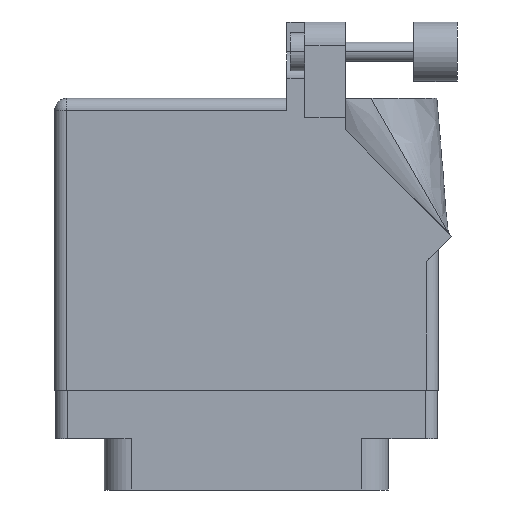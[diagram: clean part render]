
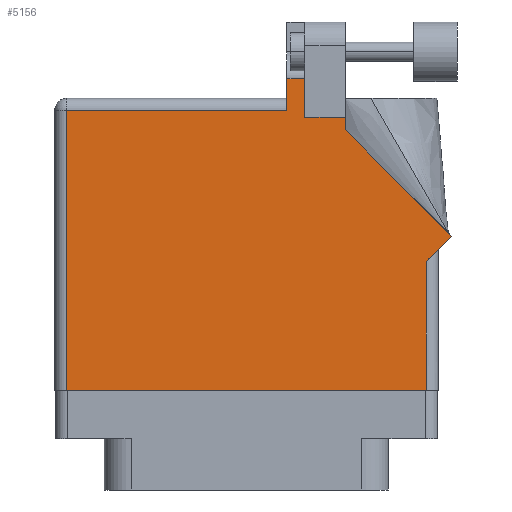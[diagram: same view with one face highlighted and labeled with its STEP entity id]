
A CAD part, front view. The second image highlights one B-rep face of the part: STEP entity #5156.
In plain terms, the highlighted face is planar.
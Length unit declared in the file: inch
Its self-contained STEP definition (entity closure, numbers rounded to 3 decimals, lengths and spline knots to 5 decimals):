
#82 = VECTOR ( 'NONE', #22160, 39.37008 ) ;
#381 = CARTESIAN_POINT ( 'NONE',  ( 0.519, 1.26442, 0.455 ) ) ;
#1623 = LINE ( 'NONE', #15452, #34094 ) ;
#1625 = CARTESIAN_POINT ( 'NONE',  ( 0.63677, 1.5315, 0.455 ) ) ;
#1646 = VECTOR ( 'NONE', #5734, 39.37008 ) ;
#2080 = VECTOR ( 'NONE', #26862, 39.37008 ) ;
#2097 = LINE ( 'NONE', #30293, #11346 ) ;
#2348 = ORIENTED_EDGE ( 'NONE', *, *, #28803, .T. ) ;
#2803 = VECTOR ( 'NONE', #6872, 39.37008 ) ;
#3260 = VECTOR ( 'NONE', #18487, 39.37008 ) ;
#3266 = VECTOR ( 'NONE', #21904, 39.37008 ) ;
#4062 = VERTEX_POINT ( 'NONE', #29323 ) ;
#4336 = VERTEX_POINT ( 'NONE', #22237 ) ;
#4407 = VERTEX_POINT ( 'NONE', #17761 ) ;
#4456 = EDGE_CURVE ( 'NONE', #25277, #4407, #30085, .T. ) ;
#4702 = ORIENTED_EDGE ( 'NONE', *, *, #26649, .T. ) ;
#5156 = ADVANCED_FACE ( 'NONE', ( #26941 ), #23604, .F. ) ;
#5289 = VERTEX_POINT ( 'NONE', #10062 ) ;
#5734 = DIRECTION ( 'NONE',  ( 0., -1., 0. ) ) ;
#6723 = DIRECTION ( 'NONE',  ( 0., 0., -1. ) ) ;
#6872 = DIRECTION ( 'NONE',  ( 0., 1., 0. ) ) ;
#6888 = LINE ( 'NONE', #381, #25368 ) ;
#7732 = EDGE_CURVE ( 'NONE', #17834, #10180, #15529, .T. ) ;
#8005 = VECTOR ( 'NONE', #28396, 39.37008 ) ;
#9336 = LINE ( 'NONE', #16384, #82 ) ;
#9558 = LINE ( 'NONE', #18669, #2080 ) ;
#9890 = EDGE_CURVE ( 'NONE', #10180, #23784, #9558, .T. ) ;
#10062 = CARTESIAN_POINT ( 'NONE',  ( 0.519, 1.26442, 0.455 ) ) ;
#10123 = EDGE_CURVE ( 'NONE', #23784, #4336, #25384, .T. ) ;
#10180 = VERTEX_POINT ( 'NONE', #11519 ) ;
#10313 = ORIENTED_EDGE ( 'NONE', *, *, #14590, .T. ) ;
#11346 = VECTOR ( 'NONE', #13627, 39.37008 ) ;
#11415 = VERTEX_POINT ( 'NONE', #34351 ) ;
#11519 = CARTESIAN_POINT ( 'NONE',  ( 0.212, 1.368, 0.455 ) ) ;
#12117 = ORIENTED_EDGE ( 'NONE', *, *, #22507, .T. ) ;
#13627 = DIRECTION ( 'NONE',  ( -1., 0., 0. ) ) ;
#14585 = CARTESIAN_POINT ( 'NONE',  ( 1.07571, 0.70771, 0.455 ) ) ;
#14590 = EDGE_CURVE ( 'NONE', #17715, #25277, #2097, .T. ) ;
#15054 = CARTESIAN_POINT ( 'NONE',  ( 1.07571, 0.70771, 0.455 ) ) ;
#15385 = DIRECTION ( 'NONE',  ( -1., 0., 0. ) ) ;
#15452 = CARTESIAN_POINT ( 'NONE',  ( -1.005, -0.1, 0.455 ) ) ;
#15529 = LINE ( 'NONE', #23043, #8005 ) ;
#16384 = CARTESIAN_POINT ( 'NONE',  ( 1.005, 0.637, 0.455 ) ) ;
#16806 = CARTESIAN_POINT ( 'NONE',  ( -0.943, 1.368, 0.455 ) ) ;
#17361 = ORIENTED_EDGE ( 'NONE', *, *, #24011, .T. ) ;
#17715 = VERTEX_POINT ( 'NONE', #21341 ) ;
#17733 = ORIENTED_EDGE ( 'NONE', *, *, #4456, .T. ) ;
#17761 = CARTESIAN_POINT ( 'NONE',  ( 0.306, 1.5315, 0.455 ) ) ;
#17834 = VERTEX_POINT ( 'NONE', #21425 ) ;
#18127 = EDGE_CURVE ( 'NONE', #11415, #4062, #33530, .T. ) ;
#18235 = DIRECTION ( 'NONE',  ( 1., 0., 0. ) ) ;
#18487 = DIRECTION ( 'NONE',  ( -1., 0., 0. ) ) ;
#18669 = CARTESIAN_POINT ( 'NONE',  ( -1.005, 1.368, 0.455 ) ) ;
#19387 = CARTESIAN_POINT ( 'NONE',  ( 0.306, 1.33, 0.455 ) ) ;
#19876 = CARTESIAN_POINT ( 'NONE',  ( -0.943, -0.1, 0.455 ) ) ;
#20693 = DIRECTION ( 'NONE',  ( -0.707, 0.707, 0. ) ) ;
#21341 = CARTESIAN_POINT ( 'NONE',  ( 0.519, 1.33, 0.455 ) ) ;
#21425 = CARTESIAN_POINT ( 'NONE',  ( 0.212, 1.5315, 0.455 ) ) ;
#21904 = DIRECTION ( 'NONE',  ( 0., 1., 0. ) ) ;
#22160 = DIRECTION ( 'NONE',  ( 0.707, 0.707, 0. ) ) ;
#22194 = LINE ( 'NONE', #1625, #3260 ) ;
#22237 = CARTESIAN_POINT ( 'NONE',  ( -0.943, -0.1, 0.455 ) ) ;
#22507 = EDGE_CURVE ( 'NONE', #4336, #11415, #1623, .T. ) ;
#22901 = DIRECTION ( 'NONE',  ( 0., 1., 0. ) ) ;
#23043 = CARTESIAN_POINT ( 'NONE',  ( 0.212, 1.43, 0.455 ) ) ;
#23127 = ORIENTED_EDGE ( 'NONE', *, *, #10123, .T. ) ;
#23495 = AXIS2_PLACEMENT_3D ( 'NONE', #29186, #6723, #15385 ) ;
#23604 = PLANE ( 'NONE',  #23495 ) ;
#23784 = VERTEX_POINT ( 'NONE', #16806 ) ;
#24011 = EDGE_CURVE ( 'NONE', #4407, #17834, #22194, .T. ) ;
#24922 = EDGE_LOOP ( 'NONE', ( #17733, #17361, #35348, #31927, #23127, #12117, #32791, #4702, #33755, #2348, #10313 ) ) ;
#25277 = VERTEX_POINT ( 'NONE', #34305 ) ;
#25368 = VECTOR ( 'NONE', #22901, 39.37008 ) ;
#25384 = LINE ( 'NONE', #19876, #1646 ) ;
#26649 = EDGE_CURVE ( 'NONE', #4062, #28212, #9336, .T. ) ;
#26862 = DIRECTION ( 'NONE',  ( -1., 0., 0. ) ) ;
#26941 = FACE_OUTER_BOUND ( 'NONE', #24922, .T. ) ;
#27160 = VECTOR ( 'NONE', #20693, 39.37008 ) ;
#28212 = VERTEX_POINT ( 'NONE', #14585 ) ;
#28396 = DIRECTION ( 'NONE',  ( 0., -1., 0. ) ) ;
#28803 = EDGE_CURVE ( 'NONE', #5289, #17715, #6888, .T. ) ;
#29186 = CARTESIAN_POINT ( 'NONE',  ( -1.005, 1.43, 0.455 ) ) ;
#29323 = CARTESIAN_POINT ( 'NONE',  ( 0.943, 0.575, 0.455 ) ) ;
#29329 = LINE ( 'NONE', #15054, #27160 ) ;
#30085 = LINE ( 'NONE', #19387, #3266 ) ;
#30293 = CARTESIAN_POINT ( 'NONE',  ( 0.519, 1.33, 0.455 ) ) ;
#31647 = CARTESIAN_POINT ( 'NONE',  ( 0.943, 0.637, 0.455 ) ) ;
#31927 = ORIENTED_EDGE ( 'NONE', *, *, #9890, .T. ) ;
#32791 = ORIENTED_EDGE ( 'NONE', *, *, #18127, .T. ) ;
#33530 = LINE ( 'NONE', #31647, #2803 ) ;
#33755 = ORIENTED_EDGE ( 'NONE', *, *, #34036, .T. ) ;
#34036 = EDGE_CURVE ( 'NONE', #28212, #5289, #29329, .T. ) ;
#34094 = VECTOR ( 'NONE', #18235, 39.37008 ) ;
#34305 = CARTESIAN_POINT ( 'NONE',  ( 0.306, 1.33, 0.455 ) ) ;
#34351 = CARTESIAN_POINT ( 'NONE',  ( 0.943, -0.1, 0.455 ) ) ;
#35348 = ORIENTED_EDGE ( 'NONE', *, *, #7732, .T. ) ;
